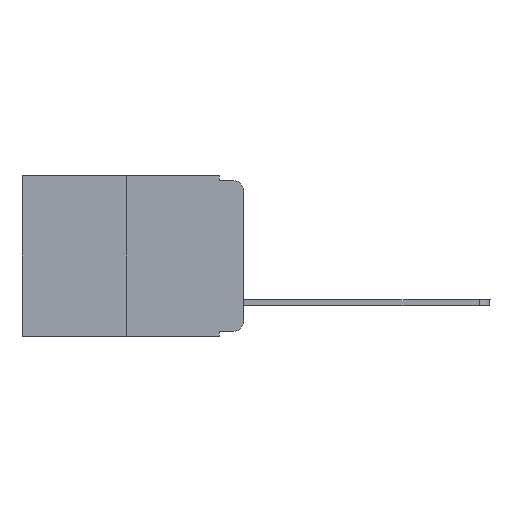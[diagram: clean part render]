
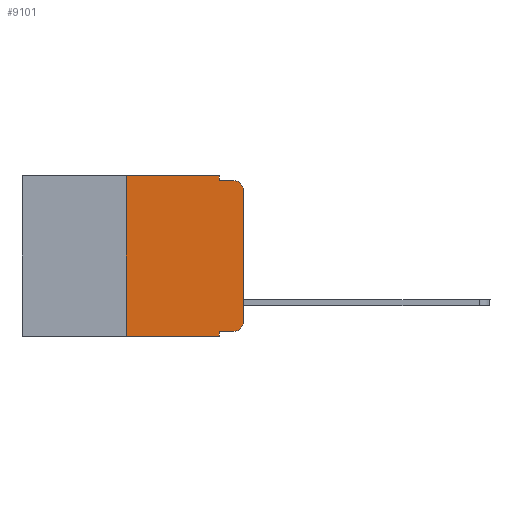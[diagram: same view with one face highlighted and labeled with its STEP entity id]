
A CAD part, left-side view. The second image highlights one B-rep face of the part: STEP entity #9101.
In plain terms, the highlighted planar face has unit normal (-1, 0, 0).
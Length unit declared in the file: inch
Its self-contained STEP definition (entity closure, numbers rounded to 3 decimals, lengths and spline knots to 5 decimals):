
#381 = CARTESIAN_POINT ( 'NONE',  ( 0., 0.25, -0.343 ) ) ;
#465 = LINE ( 'NONE', #17512, #15455 ) ;
#1180 = VECTOR ( 'NONE', #7304, 39.37008 ) ;
#1236 = CARTESIAN_POINT ( 'NONE',  ( 0., 0.051, -0.333 ) ) ;
#1448 = FACE_OUTER_BOUND ( 'NONE', #14463, .T. ) ;
#1452 = LINE ( 'NONE', #3025, #10248 ) ;
#1529 = CARTESIAN_POINT ( 'NONE',  ( 0., 0.051, -0.333 ) ) ;
#1563 = DIRECTION ( 'NONE',  ( -1., 0., 0. ) ) ;
#1988 = DIRECTION ( 'NONE',  ( 0., 0., -1. ) ) ;
#2026 = VERTEX_POINT ( 'NONE', #2069 ) ;
#2069 = CARTESIAN_POINT ( 'NONE',  ( 0., 0.051, -0.343 ) ) ;
#2210 = DIRECTION ( 'NONE',  ( -1., 0., 0. ) ) ;
#2657 = VERTEX_POINT ( 'NONE', #1236 ) ;
#3025 = CARTESIAN_POINT ( 'NONE',  ( 0., 0.051, 0. ) ) ;
#3245 = CARTESIAN_POINT ( 'NONE',  ( 0., 0.473, 0. ) ) ;
#3285 = AXIS2_PLACEMENT_3D ( 'NONE', #3245, #8356, #9803 ) ;
#3324 = EDGE_CURVE ( 'NONE', #4108, #7727, #17237, .T. ) ;
#3426 = EDGE_CURVE ( 'NONE', #7727, #9882, #6251, .T. ) ;
#4108 = VERTEX_POINT ( 'NONE', #20852 ) ;
#4460 = ORIENTED_EDGE ( 'NONE', *, *, #18665, .F. ) ;
#5102 = CARTESIAN_POINT ( 'NONE',  ( 0., 0.051, -0.01 ) ) ;
#5405 = VERTEX_POINT ( 'NONE', #10433 ) ;
#5735 = VERTEX_POINT ( 'NONE', #381 ) ;
#5966 = VECTOR ( 'NONE', #8624, 39.37008 ) ;
#6191 = VERTEX_POINT ( 'NONE', #10270 ) ;
#6228 = ORIENTED_EDGE ( 'NONE', *, *, #8805, .F. ) ;
#6251 = CIRCLE ( 'NONE', #12355, 0.02 ) ;
#6941 = CARTESIAN_POINT ( 'NONE',  ( 0., 0.051, -0.01 ) ) ;
#7121 = ORIENTED_EDGE ( 'NONE', *, *, #16792, .T. ) ;
#7304 = DIRECTION ( 'NONE',  ( 0., -1., 0. ) ) ;
#7727 = VERTEX_POINT ( 'NONE', #21526 ) ;
#8041 = DIRECTION ( 'NONE',  ( 0., 0., -1. ) ) ;
#8275 = EDGE_CURVE ( 'NONE', #2657, #5405, #14903, .T. ) ;
#8285 = LINE ( 'NONE', #15068, #14202 ) ;
#8356 = DIRECTION ( 'NONE',  ( 1., 0., 0. ) ) ;
#8379 = VECTOR ( 'NONE', #20713, 39.37008 ) ;
#8624 = DIRECTION ( 'NONE',  ( 0., -1., 0. ) ) ;
#8736 = CARTESIAN_POINT ( 'NONE',  ( 0., 0.473, -0.343 ) ) ;
#8805 = EDGE_CURVE ( 'NONE', #6191, #11966, #465, .T. ) ;
#9063 = ORIENTED_EDGE ( 'NONE', *, *, #11595, .F. ) ;
#9101 = ADVANCED_FACE ( 'NONE', ( #1448 ), #16593, .F. ) ;
#9803 = DIRECTION ( 'NONE',  ( 0., 0., -1. ) ) ;
#9882 = VERTEX_POINT ( 'NONE', #17571 ) ;
#10104 = CIRCLE ( 'NONE', #15810, 0.02 ) ;
#10248 = VECTOR ( 'NONE', #1988, 39.37008 ) ;
#10270 = CARTESIAN_POINT ( 'NONE',  ( 0., 0.051, 0. ) ) ;
#10433 = CARTESIAN_POINT ( 'NONE',  ( 0., 0.02, -0.333 ) ) ;
#10559 = DIRECTION ( 'NONE',  ( 0., 0., -1. ) ) ;
#11349 = EDGE_CURVE ( 'NONE', #5735, #13335, #16359, .T. ) ;
#11595 = EDGE_CURVE ( 'NONE', #11966, #9882, #15766, .T. ) ;
#11966 = VERTEX_POINT ( 'NONE', #6941 ) ;
#12253 = EDGE_CURVE ( 'NONE', #5405, #4108, #10104, .T. ) ;
#12355 = AXIS2_PLACEMENT_3D ( 'NONE', #14008, #2210, #10559 ) ;
#13335 = VERTEX_POINT ( 'NONE', #20485 ) ;
#13453 = DIRECTION ( 'NONE',  ( 0., -1., 0. ) ) ;
#13458 = CARTESIAN_POINT ( 'NONE',  ( 0., 0., 0. ) ) ;
#13998 = VECTOR ( 'NONE', #16685, 39.37008 ) ;
#14008 = CARTESIAN_POINT ( 'NONE',  ( 0., 0.02, -0.03 ) ) ;
#14202 = VECTOR ( 'NONE', #16851, 39.37008 ) ;
#14463 = EDGE_LOOP ( 'NONE', ( #18795, #19995, #9063, #6228, #4460, #20955, #7121, #15318, #17793, #20250 ) ) ;
#14903 = LINE ( 'NONE', #1529, #17924 ) ;
#15068 = CARTESIAN_POINT ( 'NONE',  ( 0., 0.473, 0. ) ) ;
#15318 = ORIENTED_EDGE ( 'NONE', *, *, #17779, .F. ) ;
#15455 = VECTOR ( 'NONE', #19423, 39.37008 ) ;
#15766 = LINE ( 'NONE', #5102, #1180 ) ;
#15810 = AXIS2_PLACEMENT_3D ( 'NONE', #19968, #1563, #8041 ) ;
#16359 = LINE ( 'NONE', #21736, #13998 ) ;
#16593 = PLANE ( 'NONE',  #3285 ) ;
#16685 = DIRECTION ( 'NONE',  ( 0., 0., 1. ) ) ;
#16792 = EDGE_CURVE ( 'NONE', #5735, #2026, #17093, .T. ) ;
#16851 = DIRECTION ( 'NONE',  ( 0., -1., 0. ) ) ;
#17093 = LINE ( 'NONE', #8736, #5966 ) ;
#17237 = LINE ( 'NONE', #13458, #8379 ) ;
#17512 = CARTESIAN_POINT ( 'NONE',  ( 0., 0.051, 0. ) ) ;
#17571 = CARTESIAN_POINT ( 'NONE',  ( 0., 0.02, -0.01 ) ) ;
#17779 = EDGE_CURVE ( 'NONE', #2657, #2026, #1452, .T. ) ;
#17793 = ORIENTED_EDGE ( 'NONE', *, *, #8275, .T. ) ;
#17924 = VECTOR ( 'NONE', #13453, 39.37008 ) ;
#18665 = EDGE_CURVE ( 'NONE', #13335, #6191, #8285, .T. ) ;
#18795 = ORIENTED_EDGE ( 'NONE', *, *, #3324, .T. ) ;
#19423 = DIRECTION ( 'NONE',  ( 0., 0., -1. ) ) ;
#19968 = CARTESIAN_POINT ( 'NONE',  ( 0., 0.02, -0.313 ) ) ;
#19995 = ORIENTED_EDGE ( 'NONE', *, *, #3426, .T. ) ;
#20250 = ORIENTED_EDGE ( 'NONE', *, *, #12253, .T. ) ;
#20485 = CARTESIAN_POINT ( 'NONE',  ( 0., 0.25, 0. ) ) ;
#20713 = DIRECTION ( 'NONE',  ( 0., 0., 1. ) ) ;
#20852 = CARTESIAN_POINT ( 'NONE',  ( 0., 0., -0.313 ) ) ;
#20955 = ORIENTED_EDGE ( 'NONE', *, *, #11349, .F. ) ;
#21526 = CARTESIAN_POINT ( 'NONE',  ( 0., 0., -0.03 ) ) ;
#21736 = CARTESIAN_POINT ( 'NONE',  ( 0., 0.25, 0. ) ) ;
